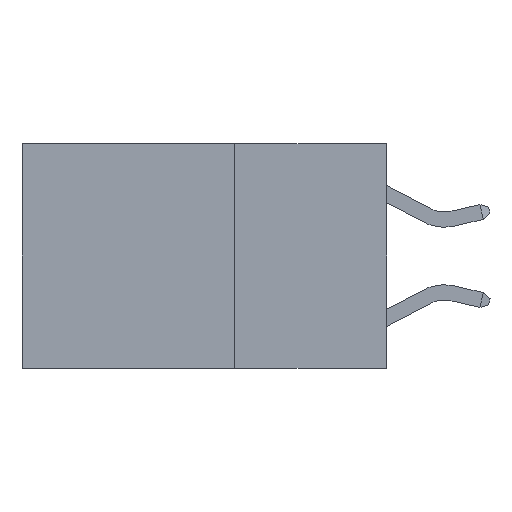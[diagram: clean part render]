
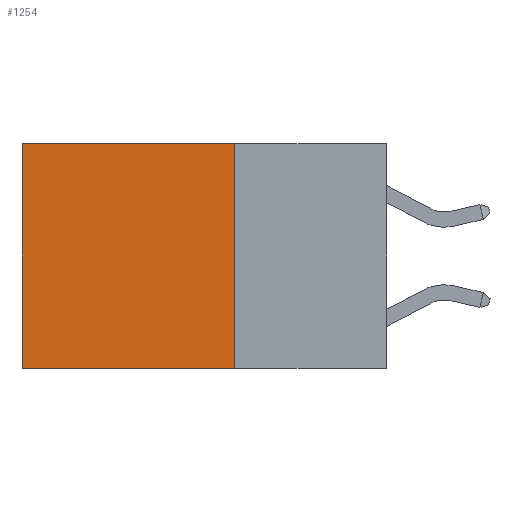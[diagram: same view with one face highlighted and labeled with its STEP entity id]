
A CAD part, left-side view. The second image highlights one B-rep face of the part: STEP entity #1254.
In plain terms, the highlighted planar face has unit normal (-1, 0, 0).
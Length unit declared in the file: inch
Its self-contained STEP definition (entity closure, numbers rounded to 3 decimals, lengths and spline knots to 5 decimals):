
#1146 = PLANE ( 'NONE',  #21004 ) ;
#1227 = EDGE_LOOP ( 'NONE', ( #22728, #3315, #10800, #4384 ) ) ;
#1254 = ADVANCED_FACE ( 'NONE', ( #25873 ), #1146, .F. ) ;
#2913 = VERTEX_POINT ( 'NONE', #9622 ) ;
#3315 = ORIENTED_EDGE ( 'NONE', *, *, #18427, .F. ) ;
#4153 = VECTOR ( 'NONE', #14860, 39.37008 ) ;
#4384 = ORIENTED_EDGE ( 'NONE', *, *, #22898, .T. ) ;
#7317 = DIRECTION ( 'NONE',  ( 0., 0., -1. ) ) ;
#7734 = VERTEX_POINT ( 'NONE', #17111 ) ;
#7865 = DIRECTION ( 'NONE',  ( 1., 0., 0. ) ) ;
#9181 = LINE ( 'NONE', #16615, #25210 ) ;
#9465 = LINE ( 'NONE', #11331, #22629 ) ;
#9622 = CARTESIAN_POINT ( 'NONE',  ( 0.2625, 0.6, -0.37 ) ) ;
#10800 = ORIENTED_EDGE ( 'NONE', *, *, #15076, .F. ) ;
#10843 = CARTESIAN_POINT ( 'NONE',  ( 0.2625, 0.25, 0. ) ) ;
#10859 = VERTEX_POINT ( 'NONE', #20307 ) ;
#11002 = DIRECTION ( 'NONE',  ( 0., 1., 0. ) ) ;
#11331 = CARTESIAN_POINT ( 'NONE',  ( 0.2625, 0.25, 0. ) ) ;
#13486 = DIRECTION ( 'NONE',  ( 0., 0., -1. ) ) ;
#14860 = DIRECTION ( 'NONE',  ( 0., 1., 0. ) ) ;
#14973 = CARTESIAN_POINT ( 'NONE',  ( 0.2625, 0.25, -0.37 ) ) ;
#15054 = EDGE_CURVE ( 'NONE', #10859, #2913, #9181, .T. ) ;
#15076 = EDGE_CURVE ( 'NONE', #7734, #24707, #9465, .T. ) ;
#16615 = CARTESIAN_POINT ( 'NONE',  ( 0.2625, 0.6, 0. ) ) ;
#17111 = CARTESIAN_POINT ( 'NONE',  ( 0.2625, 0.25, 0. ) ) ;
#17376 = DIRECTION ( 'NONE',  ( 0., 0., -1. ) ) ;
#18317 = VECTOR ( 'NONE', #11002, 39.37008 ) ;
#18427 = EDGE_CURVE ( 'NONE', #24707, #2913, #23236, .T. ) ;
#19824 = CARTESIAN_POINT ( 'NONE',  ( 0.2625, 0.25, 0. ) ) ;
#20307 = CARTESIAN_POINT ( 'NONE',  ( 0.2625, 0.6, 0. ) ) ;
#21004 = AXIS2_PLACEMENT_3D ( 'NONE', #19824, #7865, #13486 ) ;
#21201 = CARTESIAN_POINT ( 'NONE',  ( 0.2625, 0.25, -0.37 ) ) ;
#22629 = VECTOR ( 'NONE', #7317, 39.37008 ) ;
#22728 = ORIENTED_EDGE ( 'NONE', *, *, #15054, .T. ) ;
#22898 = EDGE_CURVE ( 'NONE', #7734, #10859, #25479, .T. ) ;
#23236 = LINE ( 'NONE', #21201, #18317 ) ;
#24707 = VERTEX_POINT ( 'NONE', #14973 ) ;
#25210 = VECTOR ( 'NONE', #17376, 39.37008 ) ;
#25479 = LINE ( 'NONE', #10843, #4153 ) ;
#25873 = FACE_OUTER_BOUND ( 'NONE', #1227, .T. ) ;
